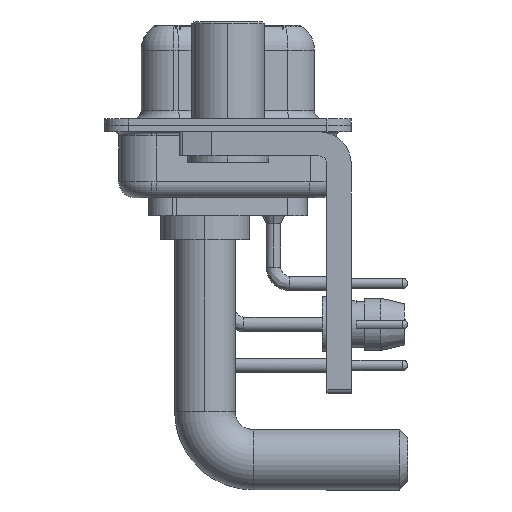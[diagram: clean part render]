
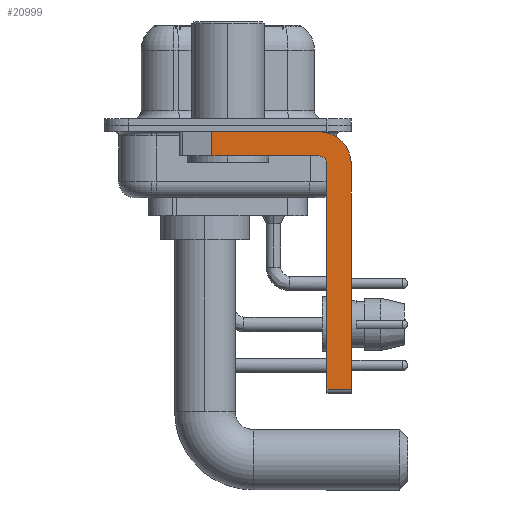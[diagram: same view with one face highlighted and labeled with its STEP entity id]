
A CAD part, left-side view. The second image highlights one B-rep face of the part: STEP entity #20999.
In plain terms, the highlighted planar face has unit normal (-1, 0, 0).
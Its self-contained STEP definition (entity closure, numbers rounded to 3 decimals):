
#1965 = CARTESIAN_POINT ( 'NONE',  ( -2.9, -7.65, -16.35 ) ) ;
#2036 = VECTOR ( 'NONE', #5491, 1000. ) ;
#2385 = CARTESIAN_POINT ( 'NONE',  ( -2.9, -5.65, -1.9 ) ) ;
#4328 = ORIENTED_EDGE ( 'NONE', *, *, #30675, .F. ) ;
#4997 = VECTOR ( 'NONE', #36588, 1000. ) ;
#5246 = EDGE_CURVE ( 'NONE', #19168, #33629, #35342, .T. ) ;
#5385 = LINE ( 'NONE', #5578, #22777 ) ;
#5491 = DIRECTION ( 'NONE',  ( 0., -1., 0. ) ) ;
#5578 = CARTESIAN_POINT ( 'NONE',  ( -2.9, -5.65, -1.9 ) ) ;
#5822 = ORIENTED_EDGE ( 'NONE', *, *, #10930, .F. ) ;
#5937 = CARTESIAN_POINT ( 'NONE',  ( -2.9, 0.978, -0.4 ) ) ;
#6053 = AXIS2_PLACEMENT_3D ( 'NONE', #13553, #25690, #10312 ) ;
#6527 = LINE ( 'NONE', #20764, #34570 ) ;
#6610 = CARTESIAN_POINT ( 'NONE',  ( -2.9, -6.15, -16.6 ) ) ;
#6794 = VERTEX_POINT ( 'NONE', #34655 ) ;
#6807 = LINE ( 'NONE', #6610, #13315 ) ;
#6990 = EDGE_CURVE ( 'NONE', #30203, #6794, #6527, .T. ) ;
#9329 = ORIENTED_EDGE ( 'NONE', *, *, #25481, .F. ) ;
#10312 = DIRECTION ( 'NONE',  ( 0., 0., -1. ) ) ;
#10930 = EDGE_CURVE ( 'NONE', #17792, #24889, #11948, .T. ) ;
#11948 = CIRCLE ( 'NONE', #20551, 2. ) ;
#12654 = CARTESIAN_POINT ( 'NONE',  ( -2.9, -6.15, -2.4 ) ) ;
#13301 = VERTEX_POINT ( 'NONE', #2385 ) ;
#13315 = VECTOR ( 'NONE', #30277, 1000. ) ;
#13553 = CARTESIAN_POINT ( 'NONE',  ( -2.9, -5.65, -2.4 ) ) ;
#14438 = DIRECTION ( 'NONE',  ( 0., 0., 1. ) ) ;
#16021 = CARTESIAN_POINT ( 'NONE',  ( -2.9, -5.65, -2.4 ) ) ;
#16586 = CARTESIAN_POINT ( 'NONE',  ( -2.9, -7.65, -2.4 ) ) ;
#17792 = VERTEX_POINT ( 'NONE', #30929 ) ;
#18625 = EDGE_CURVE ( 'NONE', #30203, #17792, #28297, .T. ) ;
#19168 = VERTEX_POINT ( 'NONE', #24965 ) ;
#19346 = FACE_OUTER_BOUND ( 'NONE', #30035, .T. ) ;
#20029 = DIRECTION ( 'NONE',  ( 1., 0., 0. ) ) ;
#20227 = VERTEX_POINT ( 'NONE', #12654 ) ;
#20551 = AXIS2_PLACEMENT_3D ( 'NONE', #37195, #20029, #22355 ) ;
#20764 = CARTESIAN_POINT ( 'NONE',  ( -2.9, 0.978, -1.9 ) ) ;
#20999 = ADVANCED_FACE ( 'NONE', ( #19346 ), #34373, .F. ) ;
#21055 = ORIENTED_EDGE ( 'NONE', *, *, #18625, .F. ) ;
#22355 = DIRECTION ( 'NONE',  ( 0., 0., -1. ) ) ;
#22500 = LINE ( 'NONE', #25576, #36460 ) ;
#22701 = CARTESIAN_POINT ( 'NONE',  ( -2.9, 3., -0.4 ) ) ;
#22777 = VECTOR ( 'NONE', #26371, 1000. ) ;
#23378 = EDGE_CURVE ( 'NONE', #13301, #6794, #5385, .T. ) ;
#24889 = VERTEX_POINT ( 'NONE', #16586 ) ;
#24959 = CIRCLE ( 'NONE', #35427, 0.5 ) ;
#24965 = CARTESIAN_POINT ( 'NONE',  ( -2.9, -6.15, -16.35 ) ) ;
#25054 = DIRECTION ( 'NONE',  ( -1., 0., 0. ) ) ;
#25184 = ORIENTED_EDGE ( 'NONE', *, *, #29609, .F. ) ;
#25481 = EDGE_CURVE ( 'NONE', #24889, #33629, #22500, .T. ) ;
#25576 = CARTESIAN_POINT ( 'NONE',  ( -2.9, -7.65, -2.4 ) ) ;
#25690 = DIRECTION ( 'NONE',  ( 1., 0., 0. ) ) ;
#25852 = ORIENTED_EDGE ( 'NONE', *, *, #23378, .F. ) ;
#26371 = DIRECTION ( 'NONE',  ( 0., 1., 0. ) ) ;
#28297 = LINE ( 'NONE', #22701, #4997 ) ;
#29551 = CARTESIAN_POINT ( 'NONE',  ( -2.9, -5.65, -16.35 ) ) ;
#29609 = EDGE_CURVE ( 'NONE', #20227, #13301, #24959, .T. ) ;
#30035 = EDGE_LOOP ( 'NONE', ( #21055, #36502, #25852, #25184, #4328, #30908, #9329, #5822 ) ) ;
#30203 = VERTEX_POINT ( 'NONE', #5937 ) ;
#30277 = DIRECTION ( 'NONE',  ( 0., 0., 1. ) ) ;
#30675 = EDGE_CURVE ( 'NONE', #19168, #20227, #6807, .T. ) ;
#30908 = ORIENTED_EDGE ( 'NONE', *, *, #5246, .T. ) ;
#30929 = CARTESIAN_POINT ( 'NONE',  ( -2.9, -5.65, -0.4 ) ) ;
#32530 = DIRECTION ( 'NONE',  ( 0., 0., -1. ) ) ;
#33629 = VERTEX_POINT ( 'NONE', #1965 ) ;
#34373 = PLANE ( 'NONE',  #6053 ) ;
#34570 = VECTOR ( 'NONE', #32530, 1000. ) ;
#34655 = CARTESIAN_POINT ( 'NONE',  ( -2.9, 0.978, -1.9 ) ) ;
#35342 = LINE ( 'NONE', #29551, #2036 ) ;
#35427 = AXIS2_PLACEMENT_3D ( 'NONE', #16021, #25054, #14438 ) ;
#36460 = VECTOR ( 'NONE', #37336, 1000. ) ;
#36502 = ORIENTED_EDGE ( 'NONE', *, *, #6990, .T. ) ;
#36588 = DIRECTION ( 'NONE',  ( 0., -1., 0. ) ) ;
#37195 = CARTESIAN_POINT ( 'NONE',  ( -2.9, -5.65, -2.4 ) ) ;
#37336 = DIRECTION ( 'NONE',  ( 0., 0., -1. ) ) ;
